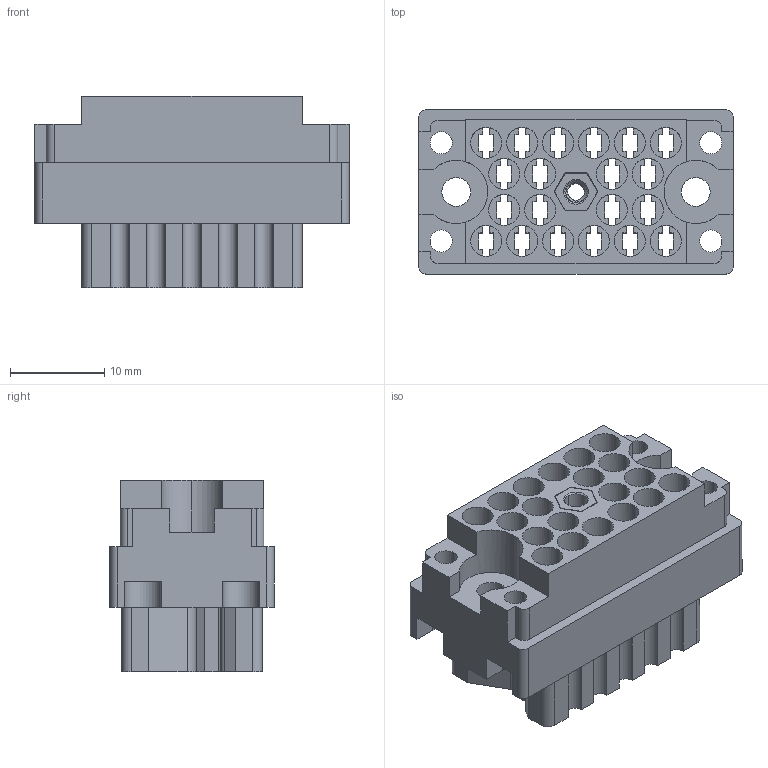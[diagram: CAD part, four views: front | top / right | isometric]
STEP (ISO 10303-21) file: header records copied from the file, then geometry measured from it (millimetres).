
FILE_DESCRIPTION (( 'STEP AP203' ), '1' );
FILE_NAME ('516-020-000-606.STEP', '2020-03-04T16:45:53', ( '' ), ( '' ), 'SwSTEP 2.0', 'SolidWorks 2016', '' );
FILE_SCHEMA (( 'CONFIG_CONTROL_DESIGN' ));
Length unit declared in the file: inch
Products named in the file (3): 516 Part Receptacle_020; 516-020-000-606; 516-252-025-100_516-252-025-100
Assembly tree (2 placements, depth 2):
  516-020-000-606
    516 Part Receptacle_020
    516-252-025-100_516-252-025-100
Bounding box: 33.32 x 17.42 x 20.27 mm (x, y, z)
Volume: 5061.5 mm3; surface area: 8513.5 mm2
Topology: 2 solids, 2 shells, 665 faces, 1937 edges, 1287 vertices
Faces by surface type: plane 424, cylinder 227, cone 11, bspline 3
Entity records: 24958 total; most frequent: CARTESIAN_POINT 6610, ORIENTED_EDGE 3874, DIRECTION 3716, EDGE_CURVE 1937, LINE 1380, VECTOR 1380, VERTEX_POINT 1287, AXIS2_PLACEMENT_3D 1168
